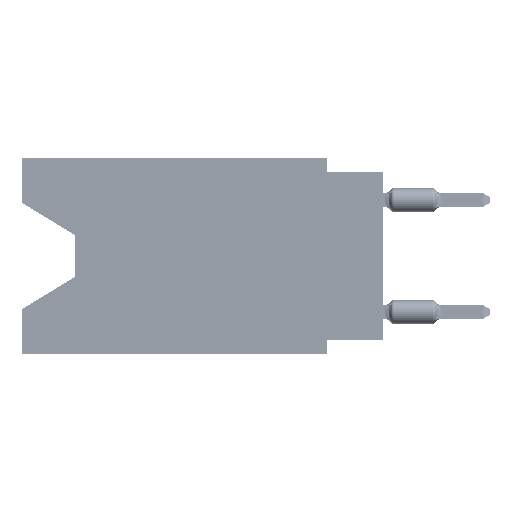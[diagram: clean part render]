
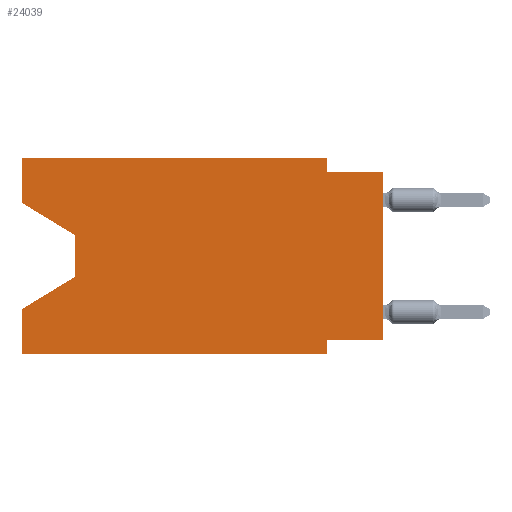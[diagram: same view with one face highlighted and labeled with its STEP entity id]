
A CAD part, left-side view. The second image highlights one B-rep face of the part: STEP entity #24039.
In plain terms, the highlighted planar face has unit normal (-1, 0, 0).
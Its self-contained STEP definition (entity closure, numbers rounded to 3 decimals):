
#160 = DIRECTION ( 'NONE',  ( 0., 0., -1. ) ) ;
#1766 = EDGE_CURVE ( 'NONE', #27214, #14664, #42431, .T. ) ;
#2174 = VERTEX_POINT ( 'NONE', #57512 ) ;
#2950 = VECTOR ( 'NONE', #42364, 1000. ) ;
#3552 = CARTESIAN_POINT ( 'NONE',  ( 0., 2.54, 0. ) ) ;
#3919 = VECTOR ( 'NONE', #65636, 1000. ) ;
#5174 = LINE ( 'NONE', #28058, #3919 ) ;
#6075 = VECTOR ( 'NONE', #51955, 1000. ) ;
#6237 = CARTESIAN_POINT ( 'NONE',  ( 0., 13.97, -3.505 ) ) ;
#7865 = CARTESIAN_POINT ( 'NONE',  ( 0., 2.54, -8.255 ) ) ;
#8737 = CARTESIAN_POINT ( 'NONE',  ( 0., 0., -8.255 ) ) ;
#8874 = LINE ( 'NONE', #14236, #23739 ) ;
#8958 = ORIENTED_EDGE ( 'NONE', *, *, #44914, .F. ) ;
#10399 = DIRECTION ( 'NONE',  ( 0., 0., 1. ) ) ;
#10754 = CARTESIAN_POINT ( 'NONE',  ( 0., 16.383, 0. ) ) ;
#10889 = VECTOR ( 'NONE', #20768, 1000. ) ;
#10915 = VERTEX_POINT ( 'NONE', #23307 ) ;
#11591 = ORIENTED_EDGE ( 'NONE', *, *, #61404, .T. ) ;
#12118 = LINE ( 'NONE', #39311, #31363 ) ;
#14236 = CARTESIAN_POINT ( 'NONE',  ( 0., 2.54, 0. ) ) ;
#14261 = CARTESIAN_POINT ( 'NONE',  ( 0., 16.383, 0. ) ) ;
#14664 = VERTEX_POINT ( 'NONE', #3552 ) ;
#14811 = LINE ( 'NONE', #8737, #2950 ) ;
#16590 = DIRECTION ( 'NONE',  ( 0., -0.855, -0.519 ) ) ;
#17124 = EDGE_CURVE ( 'NONE', #58071, #2174, #69757, .T. ) ;
#17407 = VERTEX_POINT ( 'NONE', #56823 ) ;
#17823 = EDGE_CURVE ( 'NONE', #17407, #58071, #14811, .T. ) ;
#20138 = VERTEX_POINT ( 'NONE', #58674 ) ;
#20327 = DIRECTION ( 'NONE',  ( 0., 0., -1. ) ) ;
#20768 = DIRECTION ( 'NONE',  ( 0., 0., -1. ) ) ;
#22029 = DIRECTION ( 'NONE',  ( 0., -1., 0. ) ) ;
#23307 = CARTESIAN_POINT ( 'NONE',  ( 0., 0., -0.635 ) ) ;
#23709 = LINE ( 'NONE', #50903, #6075 ) ;
#23739 = VECTOR ( 'NONE', #20327, 1000. ) ;
#23917 = ORIENTED_EDGE ( 'NONE', *, *, #41643, .F. ) ;
#24039 = ADVANCED_FACE ( 'NONE', ( #30678 ), #31391, .F. ) ;
#25667 = CARTESIAN_POINT ( 'NONE',  ( 0., 16.383, 0. ) ) ;
#26621 = LINE ( 'NONE', #55220, #67404 ) ;
#27017 = EDGE_CURVE ( 'NONE', #57013, #27214, #66189, .T. ) ;
#27214 = VERTEX_POINT ( 'NONE', #14261 ) ;
#27727 = LINE ( 'NONE', #6237, #46999 ) ;
#27998 = VERTEX_POINT ( 'NONE', #36638 ) ;
#28058 = CARTESIAN_POINT ( 'NONE',  ( 0., 0., 0. ) ) ;
#28607 = ORIENTED_EDGE ( 'NONE', *, *, #60307, .T. ) ;
#29418 = VECTOR ( 'NONE', #22029, 1000. ) ;
#30508 = CARTESIAN_POINT ( 'NONE',  ( 0., 16.383, -8.89 ) ) ;
#30678 = FACE_OUTER_BOUND ( 'NONE', #66185, .T. ) ;
#31363 = VECTOR ( 'NONE', #33942, 1000. ) ;
#31391 = PLANE ( 'NONE',  #42027 ) ;
#31983 = CARTESIAN_POINT ( 'NONE',  ( 0., 0., -0.635 ) ) ;
#32317 = ORIENTED_EDGE ( 'NONE', *, *, #55046, .T. ) ;
#33942 = DIRECTION ( 'NONE',  ( 0., 0., 1. ) ) ;
#36638 = CARTESIAN_POINT ( 'NONE',  ( 0., 13.97, -5.385 ) ) ;
#38389 = EDGE_CURVE ( 'NONE', #69676, #2174, #23709, .T. ) ;
#39267 = ORIENTED_EDGE ( 'NONE', *, *, #53836, .T. ) ;
#39311 = CARTESIAN_POINT ( 'NONE',  ( 0., 16.383, 0. ) ) ;
#39587 = ORIENTED_EDGE ( 'NONE', *, *, #27017, .F. ) ;
#39968 = VECTOR ( 'NONE', #10399, 1000. ) ;
#40142 = ORIENTED_EDGE ( 'NONE', *, *, #38389, .T. ) ;
#40913 = ORIENTED_EDGE ( 'NONE', *, *, #66357, .F. ) ;
#41643 = EDGE_CURVE ( 'NONE', #69676, #59589, #12118, .T. ) ;
#42027 = AXIS2_PLACEMENT_3D ( 'NONE', #25667, #64302, #57513 ) ;
#42088 = ORIENTED_EDGE ( 'NONE', *, *, #17823, .F. ) ;
#42364 = DIRECTION ( 'NONE',  ( 0., 1., 0. ) ) ;
#42431 = LINE ( 'NONE', #51749, #29418 ) ;
#44843 = LINE ( 'NONE', #49511, #58892 ) ;
#44914 = EDGE_CURVE ( 'NONE', #14664, #20138, #8874, .T. ) ;
#46999 = VECTOR ( 'NONE', #160, 1000. ) ;
#49511 = CARTESIAN_POINT ( 'NONE',  ( 0., 16.383, -2.038 ) ) ;
#50349 = VECTOR ( 'NONE', #65247, 1000. ) ;
#50903 = CARTESIAN_POINT ( 'NONE',  ( 0., 16.383, -8.89 ) ) ;
#51282 = CARTESIAN_POINT ( 'NONE',  ( 0., 2.54, -8.89 ) ) ;
#51749 = CARTESIAN_POINT ( 'NONE',  ( 0., 16.383, 0. ) ) ;
#51955 = DIRECTION ( 'NONE',  ( 0., -1., 0. ) ) ;
#53836 = EDGE_CURVE ( 'NONE', #27998, #59589, #26621, .T. ) ;
#54517 = LINE ( 'NONE', #31983, #50349 ) ;
#54861 = DIRECTION ( 'NONE',  ( 0., 0.855, -0.519 ) ) ;
#55046 = EDGE_CURVE ( 'NONE', #67071, #27998, #27727, .T. ) ;
#55220 = CARTESIAN_POINT ( 'NONE',  ( 0., 13.97, -5.385 ) ) ;
#56823 = CARTESIAN_POINT ( 'NONE',  ( 0., 0., -8.255 ) ) ;
#57013 = VERTEX_POINT ( 'NONE', #61075 ) ;
#57512 = CARTESIAN_POINT ( 'NONE',  ( 0., 2.54, -8.89 ) ) ;
#57513 = DIRECTION ( 'NONE',  ( 0., 0., -1. ) ) ;
#58071 = VERTEX_POINT ( 'NONE', #7865 ) ;
#58674 = CARTESIAN_POINT ( 'NONE',  ( 0., 2.54, -0.635 ) ) ;
#58892 = VECTOR ( 'NONE', #16590, 1000. ) ;
#59589 = VERTEX_POINT ( 'NONE', #67890 ) ;
#60307 = EDGE_CURVE ( 'NONE', #17407, #10915, #5174, .T. ) ;
#61075 = CARTESIAN_POINT ( 'NONE',  ( 0., 16.383, -2.038 ) ) ;
#61404 = EDGE_CURVE ( 'NONE', #57013, #67071, #44843, .T. ) ;
#63914 = CARTESIAN_POINT ( 'NONE',  ( 0., 13.97, -3.505 ) ) ;
#64302 = DIRECTION ( 'NONE',  ( 1., 0., 0. ) ) ;
#65247 = DIRECTION ( 'NONE',  ( 0., -1., 0. ) ) ;
#65636 = DIRECTION ( 'NONE',  ( 0., 0., 1. ) ) ;
#66185 = EDGE_LOOP ( 'NONE', ( #11591, #32317, #39267, #23917, #40142, #70415, #42088, #28607, #40913, #8958, #70340, #39587 ) ) ;
#66189 = LINE ( 'NONE', #10754, #39968 ) ;
#66357 = EDGE_CURVE ( 'NONE', #20138, #10915, #54517, .T. ) ;
#67071 = VERTEX_POINT ( 'NONE', #63914 ) ;
#67404 = VECTOR ( 'NONE', #54861, 1000. ) ;
#67890 = CARTESIAN_POINT ( 'NONE',  ( 0., 16.383, -6.852 ) ) ;
#69676 = VERTEX_POINT ( 'NONE', #30508 ) ;
#69757 = LINE ( 'NONE', #51282, #10889 ) ;
#70340 = ORIENTED_EDGE ( 'NONE', *, *, #1766, .F. ) ;
#70415 = ORIENTED_EDGE ( 'NONE', *, *, #17124, .F. ) ;
